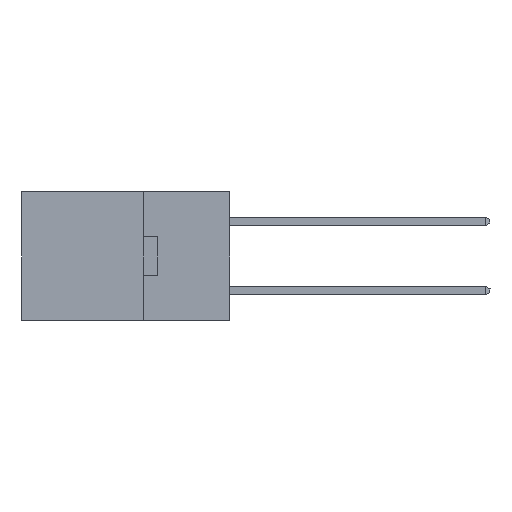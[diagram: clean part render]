
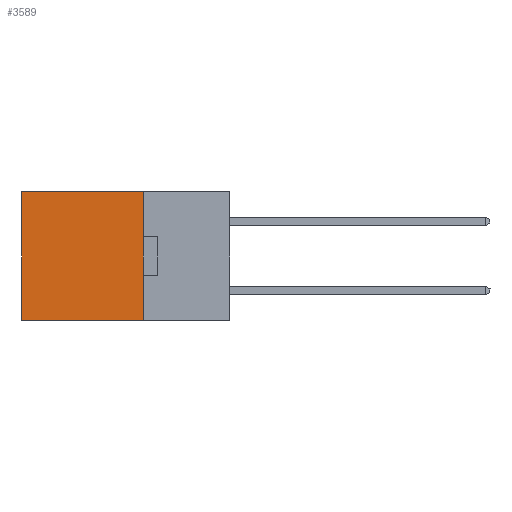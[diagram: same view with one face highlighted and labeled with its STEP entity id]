
A CAD part, left-side view. The second image highlights one B-rep face of the part: STEP entity #3589.
In plain terms, the highlighted planar face has unit normal (-1, 0, 0).
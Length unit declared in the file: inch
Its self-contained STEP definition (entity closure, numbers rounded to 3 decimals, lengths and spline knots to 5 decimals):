
#983 = VERTEX_POINT ( 'NONE', #21252 ) ;
#3292 = AXIS2_PLACEMENT_3D ( 'NONE', #14942, #19349, #5981 ) ;
#3589 = ADVANCED_FACE ( 'NONE', ( #12615 ), #3713, .F. ) ;
#3713 = PLANE ( 'NONE',  #3292 ) ;
#3793 = CARTESIAN_POINT ( 'NONE',  ( 0.2615, 0.25, -0.37 ) ) ;
#4917 = LINE ( 'NONE', #8475, #16835 ) ;
#5981 = DIRECTION ( 'NONE',  ( 0., 0., -1. ) ) ;
#6054 = DIRECTION ( 'NONE',  ( 0., 1., 0. ) ) ;
#6944 = VERTEX_POINT ( 'NONE', #17565 ) ;
#8041 = VERTEX_POINT ( 'NONE', #16818 ) ;
#8475 = CARTESIAN_POINT ( 'NONE',  ( 0.2615, 0.25, 0. ) ) ;
#8576 = LINE ( 'NONE', #3793, #19748 ) ;
#8734 = ORIENTED_EDGE ( 'NONE', *, *, #21050, .F. ) ;
#10516 = CARTESIAN_POINT ( 'NONE',  ( 0.2615, 0.25, -0.37 ) ) ;
#12615 = FACE_OUTER_BOUND ( 'NONE', #12737, .T. ) ;
#12671 = CARTESIAN_POINT ( 'NONE',  ( 0.2615, 0.6, -0.37 ) ) ;
#12717 = CARTESIAN_POINT ( 'NONE',  ( 0.2615, 0.25, 0. ) ) ;
#12737 = EDGE_LOOP ( 'NONE', ( #22201, #17388, #8734, #18193 ) ) ;
#14925 = DIRECTION ( 'NONE',  ( 0., 0., -1. ) ) ;
#14942 = CARTESIAN_POINT ( 'NONE',  ( 0.2615, 0.25, -0.37 ) ) ;
#15304 = VECTOR ( 'NONE', #14925, 39.37008 ) ;
#15782 = EDGE_CURVE ( 'NONE', #983, #6944, #26920, .T. ) ;
#15825 = EDGE_CURVE ( 'NONE', #8041, #6944, #8576, .T. ) ;
#16818 = CARTESIAN_POINT ( 'NONE',  ( 0.2615, 0.25, -0.37 ) ) ;
#16835 = VECTOR ( 'NONE', #23977, 39.37008 ) ;
#17155 = VECTOR ( 'NONE', #23756, 39.37008 ) ;
#17388 = ORIENTED_EDGE ( 'NONE', *, *, #15825, .F. ) ;
#17565 = CARTESIAN_POINT ( 'NONE',  ( 0.2615, 0.6, -0.37 ) ) ;
#18193 = ORIENTED_EDGE ( 'NONE', *, *, #20396, .T. ) ;
#19349 = DIRECTION ( 'NONE',  ( 1., 0., 0. ) ) ;
#19748 = VECTOR ( 'NONE', #6054, 39.37008 ) ;
#20396 = EDGE_CURVE ( 'NONE', #23304, #983, #4917, .T. ) ;
#21050 = EDGE_CURVE ( 'NONE', #23304, #8041, #28749, .T. ) ;
#21252 = CARTESIAN_POINT ( 'NONE',  ( 0.2615, 0.6, 0. ) ) ;
#22201 = ORIENTED_EDGE ( 'NONE', *, *, #15782, .T. ) ;
#23304 = VERTEX_POINT ( 'NONE', #12717 ) ;
#23756 = DIRECTION ( 'NONE',  ( 0., 0., -1. ) ) ;
#23977 = DIRECTION ( 'NONE',  ( 0., 1., 0. ) ) ;
#26920 = LINE ( 'NONE', #12671, #15304 ) ;
#28749 = LINE ( 'NONE', #10516, #17155 ) ;
